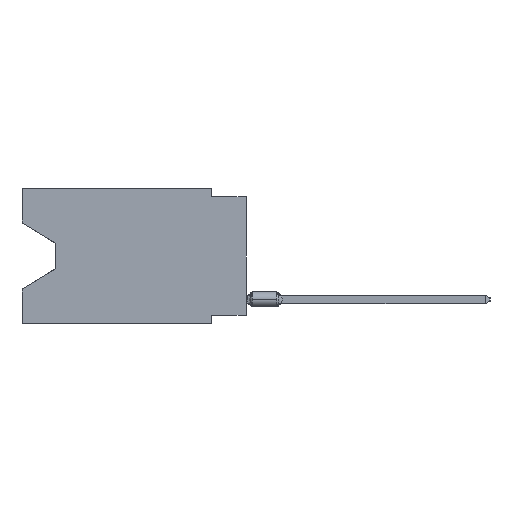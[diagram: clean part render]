
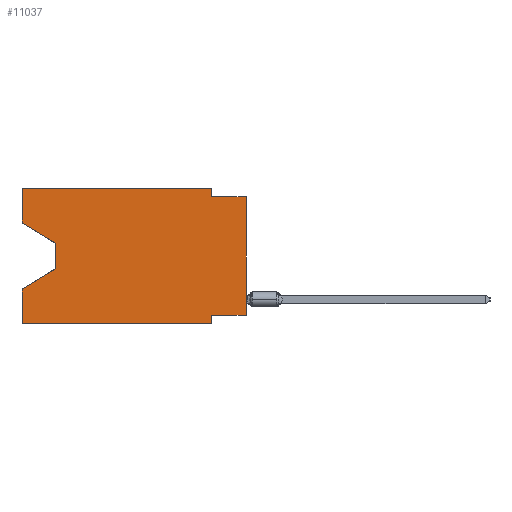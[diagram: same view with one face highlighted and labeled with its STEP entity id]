
A CAD part, left-side view. The second image highlights one B-rep face of the part: STEP entity #11037.
In plain terms, the highlighted planar face has unit normal (-1, 0, 0).
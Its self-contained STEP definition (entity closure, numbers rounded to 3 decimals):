
#661 = CARTESIAN_POINT ( 'NONE',  ( 0., 16.383, 0. ) ) ;
#827 = CARTESIAN_POINT ( 'NONE',  ( 0., 13.97, -5.893 ) ) ;
#900 = LINE ( 'NONE', #661, #22999 ) ;
#1307 = VECTOR ( 'NONE', #39575, 1000. ) ;
#1593 = ORIENTED_EDGE ( 'NONE', *, *, #34621, .T. ) ;
#1953 = EDGE_CURVE ( 'NONE', #9010, #17383, #47303, .T. ) ;
#3050 = LINE ( 'NONE', #25580, #1307 ) ;
#3155 = EDGE_CURVE ( 'NONE', #34841, #4015, #24339, .T. ) ;
#3472 = CARTESIAN_POINT ( 'NONE',  ( 0., 16.383, 0. ) ) ;
#4015 = VERTEX_POINT ( 'NONE', #44064 ) ;
#4460 = VECTOR ( 'NONE', #37492, 1000. ) ;
#5662 = DIRECTION ( 'NONE',  ( 0., 0., -1. ) ) ;
#5760 = CARTESIAN_POINT ( 'NONE',  ( 0., 0., 0. ) ) ;
#5919 = DIRECTION ( 'NONE',  ( 0., 0.855, -0.519 ) ) ;
#6188 = VERTEX_POINT ( 'NONE', #32842 ) ;
#6348 = VECTOR ( 'NONE', #32627, 1000. ) ;
#6633 = CARTESIAN_POINT ( 'NONE',  ( 0., 16.383, 0. ) ) ;
#7152 = VECTOR ( 'NONE', #14343, 1000. ) ;
#7433 = ORIENTED_EDGE ( 'NONE', *, *, #22028, .F. ) ;
#7774 = CARTESIAN_POINT ( 'NONE',  ( 0., 2.54, -9.271 ) ) ;
#7859 = VERTEX_POINT ( 'NONE', #827 ) ;
#8110 = VERTEX_POINT ( 'NONE', #22516 ) ;
#8640 = EDGE_CURVE ( 'NONE', #25443, #6188, #3050, .T. ) ;
#8799 = VECTOR ( 'NONE', #21365, 1000. ) ;
#9010 = VERTEX_POINT ( 'NONE', #31688 ) ;
#9465 = ORIENTED_EDGE ( 'NONE', *, *, #18816, .T. ) ;
#9594 = ORIENTED_EDGE ( 'NONE', *, *, #45822, .T. ) ;
#9649 = DIRECTION ( 'NONE',  ( 0., 1., 0. ) ) ;
#9838 = LINE ( 'NONE', #44141, #48259 ) ;
#9904 = LINE ( 'NONE', #43725, #46760 ) ;
#9992 = EDGE_LOOP ( 'NONE', ( #10579, #9594, #9465, #12941, #41845, #34013, #45567, #1593, #7433, #36427, #39732, #42723 ) ) ;
#10579 = ORIENTED_EDGE ( 'NONE', *, *, #19632, .T. ) ;
#11037 = ADVANCED_FACE ( 'NONE', ( #15879 ), #37443, .F. ) ;
#11276 = LINE ( 'NONE', #37241, #4460 ) ;
#12941 = ORIENTED_EDGE ( 'NONE', *, *, #35540, .F. ) ;
#13561 = CARTESIAN_POINT ( 'NONE',  ( 0., 16.383, -9.906 ) ) ;
#14092 = LINE ( 'NONE', #5760, #7152 ) ;
#14343 = DIRECTION ( 'NONE',  ( 0., 0., 1. ) ) ;
#14992 = CARTESIAN_POINT ( 'NONE',  ( 0., 16.383, 0. ) ) ;
#15614 = DIRECTION ( 'NONE',  ( 0., 0., 1. ) ) ;
#15777 = EDGE_CURVE ( 'NONE', #35858, #40023, #43228, .T. ) ;
#15879 = FACE_OUTER_BOUND ( 'NONE', #9992, .T. ) ;
#17251 = VERTEX_POINT ( 'NONE', #42697 ) ;
#17383 = VERTEX_POINT ( 'NONE', #14992 ) ;
#18722 = CARTESIAN_POINT ( 'NONE',  ( 0., 0., -0.635 ) ) ;
#18816 = EDGE_CURVE ( 'NONE', #7859, #36275, #9838, .T. ) ;
#19632 = EDGE_CURVE ( 'NONE', #9010, #17251, #9904, .T. ) ;
#19926 = VECTOR ( 'NONE', #9649, 1000. ) ;
#20447 = CARTESIAN_POINT ( 'NONE',  ( 0., 0., -9.271 ) ) ;
#20666 = DIRECTION ( 'NONE',  ( 0., -1., 0. ) ) ;
#21365 = DIRECTION ( 'NONE',  ( 0., -1., 0. ) ) ;
#22028 = EDGE_CURVE ( 'NONE', #6188, #8110, #45169, .T. ) ;
#22246 = CARTESIAN_POINT ( 'NONE',  ( 0., 16.383, 0. ) ) ;
#22516 = CARTESIAN_POINT ( 'NONE',  ( 0., 0., -0.635 ) ) ;
#22600 = VECTOR ( 'NONE', #30234, 1000. ) ;
#22999 = VECTOR ( 'NONE', #15614, 1000. ) ;
#24281 = LINE ( 'NONE', #28915, #35716 ) ;
#24339 = LINE ( 'NONE', #13561, #35288 ) ;
#24847 = DIRECTION ( 'NONE',  ( 0., -0.855, -0.519 ) ) ;
#25443 = VERTEX_POINT ( 'NONE', #25632 ) ;
#25580 = CARTESIAN_POINT ( 'NONE',  ( 0., 2.54, 0. ) ) ;
#25632 = CARTESIAN_POINT ( 'NONE',  ( 0., 2.54, 0. ) ) ;
#28915 = CARTESIAN_POINT ( 'NONE',  ( 0., 13.97, -4.013 ) ) ;
#30234 = DIRECTION ( 'NONE',  ( 0., -1., 0. ) ) ;
#31688 = CARTESIAN_POINT ( 'NONE',  ( 0., 16.383, -2.546 ) ) ;
#32627 = DIRECTION ( 'NONE',  ( 0., 0., 1. ) ) ;
#32842 = CARTESIAN_POINT ( 'NONE',  ( 0., 2.54, -0.635 ) ) ;
#33142 = CARTESIAN_POINT ( 'NONE',  ( 0., 16.383, -7.36 ) ) ;
#33928 = CARTESIAN_POINT ( 'NONE',  ( 0., 0., -9.271 ) ) ;
#34013 = ORIENTED_EDGE ( 'NONE', *, *, #45990, .F. ) ;
#34621 = EDGE_CURVE ( 'NONE', #35858, #8110, #14092, .T. ) ;
#34841 = VERTEX_POINT ( 'NONE', #35365 ) ;
#35288 = VECTOR ( 'NONE', #20666, 1000. ) ;
#35365 = CARTESIAN_POINT ( 'NONE',  ( 0., 16.383, -9.906 ) ) ;
#35540 = EDGE_CURVE ( 'NONE', #34841, #36275, #900, .T. ) ;
#35716 = VECTOR ( 'NONE', #5662, 1000. ) ;
#35858 = VERTEX_POINT ( 'NONE', #33928 ) ;
#36275 = VERTEX_POINT ( 'NONE', #33142 ) ;
#36427 = ORIENTED_EDGE ( 'NONE', *, *, #8640, .F. ) ;
#37241 = CARTESIAN_POINT ( 'NONE',  ( 0., 2.54, -9.906 ) ) ;
#37443 = PLANE ( 'NONE',  #44466 ) ;
#37492 = DIRECTION ( 'NONE',  ( 0., 0., -1. ) ) ;
#37688 = DIRECTION ( 'NONE',  ( 1., 0., 0. ) ) ;
#39575 = DIRECTION ( 'NONE',  ( 0., 0., -1. ) ) ;
#39732 = ORIENTED_EDGE ( 'NONE', *, *, #43440, .F. ) ;
#40023 = VERTEX_POINT ( 'NONE', #7774 ) ;
#41839 = DIRECTION ( 'NONE',  ( 0., 0., -1. ) ) ;
#41845 = ORIENTED_EDGE ( 'NONE', *, *, #3155, .T. ) ;
#42697 = CARTESIAN_POINT ( 'NONE',  ( 0., 13.97, -4.013 ) ) ;
#42723 = ORIENTED_EDGE ( 'NONE', *, *, #1953, .F. ) ;
#43228 = LINE ( 'NONE', #20447, #19926 ) ;
#43440 = EDGE_CURVE ( 'NONE', #17383, #25443, #47563, .T. ) ;
#43725 = CARTESIAN_POINT ( 'NONE',  ( 0., 16.383, -2.546 ) ) ;
#44064 = CARTESIAN_POINT ( 'NONE',  ( 0., 2.54, -9.906 ) ) ;
#44141 = CARTESIAN_POINT ( 'NONE',  ( 0., 13.97, -5.893 ) ) ;
#44466 = AXIS2_PLACEMENT_3D ( 'NONE', #22246, #37688, #41839 ) ;
#45169 = LINE ( 'NONE', #18722, #22600 ) ;
#45567 = ORIENTED_EDGE ( 'NONE', *, *, #15777, .F. ) ;
#45822 = EDGE_CURVE ( 'NONE', #17251, #7859, #24281, .T. ) ;
#45990 = EDGE_CURVE ( 'NONE', #40023, #4015, #11276, .T. ) ;
#46760 = VECTOR ( 'NONE', #24847, 1000. ) ;
#47303 = LINE ( 'NONE', #6633, #6348 ) ;
#47563 = LINE ( 'NONE', #3472, #8799 ) ;
#48259 = VECTOR ( 'NONE', #5919, 1000. ) ;
